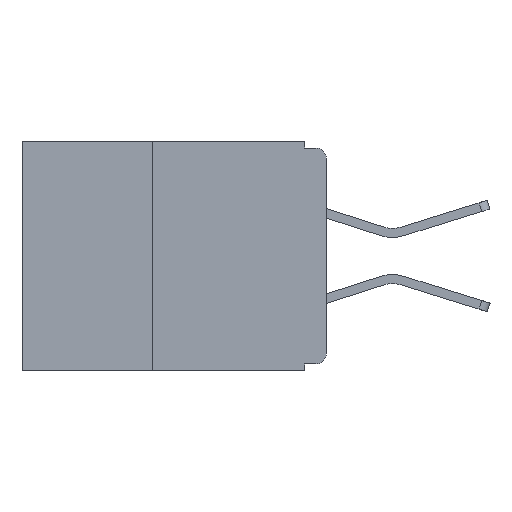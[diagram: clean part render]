
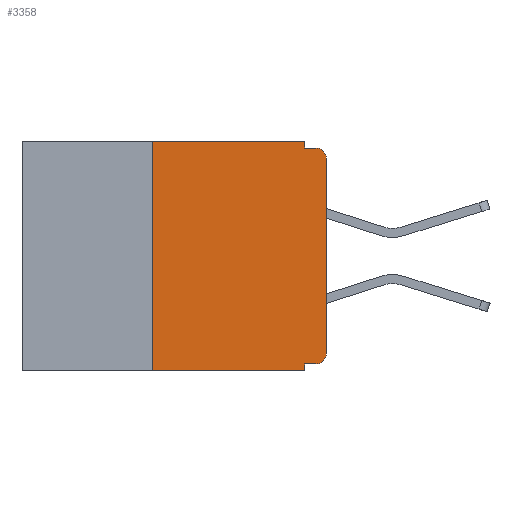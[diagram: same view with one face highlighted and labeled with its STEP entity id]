
A CAD part, left-side view. The second image highlights one B-rep face of the part: STEP entity #3358.
In plain terms, the highlighted planar face has unit normal (-1, 0, 0).
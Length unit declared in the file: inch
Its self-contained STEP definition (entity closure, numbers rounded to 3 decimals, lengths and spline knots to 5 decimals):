
#396 = DIRECTION ( 'NONE',  ( 0., 0., -1. ) ) ;
#481 = VERTEX_POINT ( 'NONE', #11794 ) ;
#640 = ORIENTED_EDGE ( 'NONE', *, *, #13596, .F. ) ;
#871 = VERTEX_POINT ( 'NONE', #7934 ) ;
#1219 = CARTESIAN_POINT ( 'NONE',  ( 0., 0.031, -0.33 ) ) ;
#1291 = LINE ( 'NONE', #8791, #17403 ) ;
#1347 = EDGE_CURVE ( 'NONE', #9917, #18571, #1291, .T. ) ;
#1979 = DIRECTION ( 'NONE',  ( 0., -1., 0. ) ) ;
#2388 = LINE ( 'NONE', #16566, #7021 ) ;
#2689 = LINE ( 'NONE', #8220, #5831 ) ;
#2890 = LINE ( 'NONE', #4273, #18955 ) ;
#3358 = ADVANCED_FACE ( 'NONE', ( #8621 ), #17765, .F. ) ;
#3651 = CARTESIAN_POINT ( 'NONE',  ( 0., 0.031, 0. ) ) ;
#3778 = VERTEX_POINT ( 'NONE', #5215 ) ;
#3840 = LINE ( 'NONE', #5154, #19875 ) ;
#4273 = CARTESIAN_POINT ( 'NONE',  ( 0., 0.437, -0.33 ) ) ;
#4339 = VECTOR ( 'NONE', #16140, 39.37008 ) ;
#4351 = CIRCLE ( 'NONE', #7969, 0.015 ) ;
#4381 = DIRECTION ( 'NONE',  ( -1., 0., 0. ) ) ;
#5154 = CARTESIAN_POINT ( 'NONE',  ( 0., 0., 0. ) ) ;
#5215 = CARTESIAN_POINT ( 'NONE',  ( 0., 0.25, -0.33 ) ) ;
#5510 = EDGE_CURVE ( 'NONE', #18018, #18187, #15283, .T. ) ;
#5831 = VECTOR ( 'NONE', #1979, 39.37008 ) ;
#7021 = VECTOR ( 'NONE', #11910, 39.37008 ) ;
#7194 = DIRECTION ( 'NONE',  ( 0., 0., -1. ) ) ;
#7217 = DIRECTION ( 'NONE',  ( 1., 0., 0. ) ) ;
#7738 = DIRECTION ( 'NONE',  ( -1., 0., 0. ) ) ;
#7934 = CARTESIAN_POINT ( 'NONE',  ( 0., 0., -0.025 ) ) ;
#7969 = AXIS2_PLACEMENT_3D ( 'NONE', #17040, #7738, #18557 ) ;
#8219 = VECTOR ( 'NONE', #396, 39.37008 ) ;
#8220 = CARTESIAN_POINT ( 'NONE',  ( 0., 0., -0.01 ) ) ;
#8225 = ORIENTED_EDGE ( 'NONE', *, *, #19254, .F. ) ;
#8621 = FACE_OUTER_BOUND ( 'NONE', #15116, .T. ) ;
#8692 = ORIENTED_EDGE ( 'NONE', *, *, #1347, .F. ) ;
#8702 = DIRECTION ( 'NONE',  ( 0., 1., 0. ) ) ;
#8781 = CARTESIAN_POINT ( 'NONE',  ( 0., 0.031, -0.32 ) ) ;
#8791 = CARTESIAN_POINT ( 'NONE',  ( 0., 0., -0.32 ) ) ;
#9019 = DIRECTION ( 'NONE',  ( 0., -1., 0. ) ) ;
#9246 = EDGE_CURVE ( 'NONE', #871, #481, #4351, .T. ) ;
#9872 = DIRECTION ( 'NONE',  ( 0., -1., 0. ) ) ;
#9917 = VERTEX_POINT ( 'NONE', #11229 ) ;
#10171 = AXIS2_PLACEMENT_3D ( 'NONE', #13779, #4381, #15322 ) ;
#10444 = CARTESIAN_POINT ( 'NONE',  ( 0., 0.25, 0. ) ) ;
#10758 = ORIENTED_EDGE ( 'NONE', *, *, #14743, .T. ) ;
#11229 = CARTESIAN_POINT ( 'NONE',  ( 0., 0.015, -0.32 ) ) ;
#11626 = ORIENTED_EDGE ( 'NONE', *, *, #15539, .T. ) ;
#11794 = CARTESIAN_POINT ( 'NONE',  ( 0., 0.015, -0.01 ) ) ;
#11910 = DIRECTION ( 'NONE',  ( 0., 0., 1. ) ) ;
#12377 = LINE ( 'NONE', #17517, #8219 ) ;
#13249 = EDGE_CURVE ( 'NONE', #3778, #14419, #2890, .T. ) ;
#13596 = EDGE_CURVE ( 'NONE', #18187, #19407, #16314, .T. ) ;
#13779 = CARTESIAN_POINT ( 'NONE',  ( 0., 0.015, -0.305 ) ) ;
#14100 = CARTESIAN_POINT ( 'NONE',  ( 0., 0., -0.305 ) ) ;
#14119 = CIRCLE ( 'NONE', #10171, 0.015 ) ;
#14419 = VERTEX_POINT ( 'NONE', #1219 ) ;
#14578 = DIRECTION ( 'NONE',  ( 0., 0., 1. ) ) ;
#14743 = EDGE_CURVE ( 'NONE', #16324, #871, #3840, .T. ) ;
#14806 = VECTOR ( 'NONE', #9872, 39.37008 ) ;
#15116 = EDGE_LOOP ( 'NONE', ( #10758, #17281, #15620, #640, #16618, #8225, #19911, #16981, #8692, #11626 ) ) ;
#15283 = LINE ( 'NONE', #19038, #14806 ) ;
#15322 = DIRECTION ( 'NONE',  ( 0., 0., -1. ) ) ;
#15539 = EDGE_CURVE ( 'NONE', #9917, #16324, #14119, .T. ) ;
#15606 = CARTESIAN_POINT ( 'NONE',  ( 0., 0.031, 0. ) ) ;
#15620 = ORIENTED_EDGE ( 'NONE', *, *, #17747, .F. ) ;
#15826 = EDGE_CURVE ( 'NONE', #18571, #14419, #12377, .T. ) ;
#16140 = DIRECTION ( 'NONE',  ( 0., 0., -1. ) ) ;
#16314 = LINE ( 'NONE', #3651, #4339 ) ;
#16324 = VERTEX_POINT ( 'NONE', #14100 ) ;
#16566 = CARTESIAN_POINT ( 'NONE',  ( 0., 0.25, -0.33 ) ) ;
#16618 = ORIENTED_EDGE ( 'NONE', *, *, #5510, .F. ) ;
#16890 = CARTESIAN_POINT ( 'NONE',  ( 0., 0.031, -0.01 ) ) ;
#16981 = ORIENTED_EDGE ( 'NONE', *, *, #15826, .F. ) ;
#17040 = CARTESIAN_POINT ( 'NONE',  ( 0., 0.015, -0.025 ) ) ;
#17118 = AXIS2_PLACEMENT_3D ( 'NONE', #17781, #7217, #7194 ) ;
#17281 = ORIENTED_EDGE ( 'NONE', *, *, #9246, .T. ) ;
#17403 = VECTOR ( 'NONE', #8702, 39.37008 ) ;
#17517 = CARTESIAN_POINT ( 'NONE',  ( 0., 0.031, -0.33 ) ) ;
#17747 = EDGE_CURVE ( 'NONE', #19407, #481, #2689, .T. ) ;
#17765 = PLANE ( 'NONE',  #17118 ) ;
#17781 = CARTESIAN_POINT ( 'NONE',  ( 0., 0.437, 0. ) ) ;
#18018 = VERTEX_POINT ( 'NONE', #10444 ) ;
#18187 = VERTEX_POINT ( 'NONE', #15606 ) ;
#18557 = DIRECTION ( 'NONE',  ( 0., 0., -1. ) ) ;
#18571 = VERTEX_POINT ( 'NONE', #8781 ) ;
#18955 = VECTOR ( 'NONE', #9019, 39.37008 ) ;
#19038 = CARTESIAN_POINT ( 'NONE',  ( 0., 0.437, 0. ) ) ;
#19254 = EDGE_CURVE ( 'NONE', #3778, #18018, #2388, .T. ) ;
#19407 = VERTEX_POINT ( 'NONE', #16890 ) ;
#19875 = VECTOR ( 'NONE', #14578, 39.37008 ) ;
#19911 = ORIENTED_EDGE ( 'NONE', *, *, #13249, .T. ) ;
